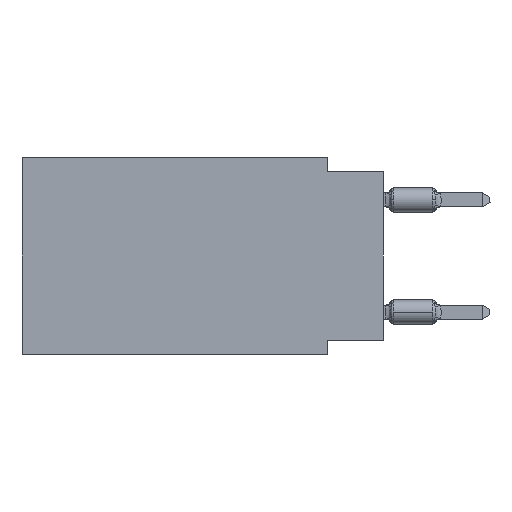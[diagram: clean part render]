
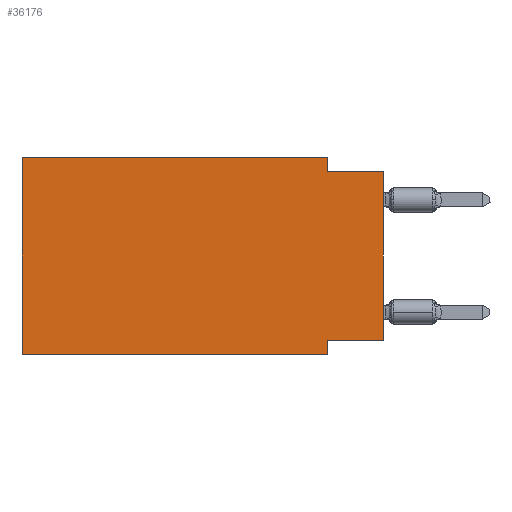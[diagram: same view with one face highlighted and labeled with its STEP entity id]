
A CAD part, left-side view. The second image highlights one B-rep face of the part: STEP entity #36176.
In plain terms, the highlighted planar face has unit normal (-1, 0, 0).
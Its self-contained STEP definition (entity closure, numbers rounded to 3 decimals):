
#5081 = CARTESIAN_POINT ( 'NONE',  ( 0., 0., -0.635 ) ) ;
#5878 = LINE ( 'NONE', #24219, #39265 ) ;
#6838 = VECTOR ( 'NONE', #38249, 1000. ) ;
#7931 = CARTESIAN_POINT ( 'NONE',  ( 0., 2.54, 0. ) ) ;
#9009 = EDGE_CURVE ( 'NONE', #35786, #32099, #42943, .T. ) ;
#9018 = VECTOR ( 'NONE', #39912, 1000. ) ;
#9441 = VERTEX_POINT ( 'NONE', #12485 ) ;
#9803 = AXIS2_PLACEMENT_3D ( 'NONE', #36194, #58762, #30806 ) ;
#11389 = DIRECTION ( 'NONE',  ( 0., 0., 1. ) ) ;
#11688 = CARTESIAN_POINT ( 'NONE',  ( 0., 0., -8.255 ) ) ;
#12299 = ORIENTED_EDGE ( 'NONE', *, *, #9009, .T. ) ;
#12485 = CARTESIAN_POINT ( 'NONE',  ( 0., 2.54, -0.635 ) ) ;
#12638 = CARTESIAN_POINT ( 'NONE',  ( 0., 0., -8.255 ) ) ;
#14090 = EDGE_CURVE ( 'NONE', #54778, #34533, #27124, .T. ) ;
#14154 = EDGE_CURVE ( 'NONE', #33876, #26621, #50866, .T. ) ;
#15333 = CARTESIAN_POINT ( 'NONE',  ( 0., 2.54, -8.89 ) ) ;
#15729 = VECTOR ( 'NONE', #11389, 1000. ) ;
#15872 = VECTOR ( 'NONE', #42698, 1000. ) ;
#16731 = EDGE_CURVE ( 'NONE', #40466, #9441, #20872, .T. ) ;
#17836 = EDGE_CURVE ( 'NONE', #26621, #40466, #5878, .T. ) ;
#18062 = VECTOR ( 'NONE', #42431, 1000. ) ;
#18704 = EDGE_CURVE ( 'NONE', #33876, #34533, #46908, .T. ) ;
#19930 = CARTESIAN_POINT ( 'NONE',  ( 0., 0., -0.635 ) ) ;
#20116 = CARTESIAN_POINT ( 'NONE',  ( 0., 0., 0. ) ) ;
#20848 = ORIENTED_EDGE ( 'NONE', *, *, #53926, .F. ) ;
#20872 = LINE ( 'NONE', #7931, #47003 ) ;
#21926 = ORIENTED_EDGE ( 'NONE', *, *, #45722, .F. ) ;
#22688 = CARTESIAN_POINT ( 'NONE',  ( 0., 2.54, -8.255 ) ) ;
#24219 = CARTESIAN_POINT ( 'NONE',  ( 0., 16.383, 0. ) ) ;
#25162 = ORIENTED_EDGE ( 'NONE', *, *, #14090, .F. ) ;
#26089 = ORIENTED_EDGE ( 'NONE', *, *, #17836, .F. ) ;
#26518 = CARTESIAN_POINT ( 'NONE',  ( 0., 2.54, -8.89 ) ) ;
#26621 = VERTEX_POINT ( 'NONE', #32215 ) ;
#27124 = LINE ( 'NONE', #26518, #52612 ) ;
#29075 = ORIENTED_EDGE ( 'NONE', *, *, #16731, .F. ) ;
#30806 = DIRECTION ( 'NONE',  ( 0., 0., -1. ) ) ;
#31397 = PLANE ( 'NONE',  #9803 ) ;
#32099 = VERTEX_POINT ( 'NONE', #5081 ) ;
#32215 = CARTESIAN_POINT ( 'NONE',  ( 0., 16.383, 0. ) ) ;
#33876 = VERTEX_POINT ( 'NONE', #42848 ) ;
#34533 = VERTEX_POINT ( 'NONE', #15333 ) ;
#35786 = VERTEX_POINT ( 'NONE', #12638 ) ;
#36176 = ADVANCED_FACE ( 'NONE', ( #44918 ), #31397, .F. ) ;
#36194 = CARTESIAN_POINT ( 'NONE',  ( 0., 16.383, 0. ) ) ;
#36410 = DIRECTION ( 'NONE',  ( 0., 0., -1. ) ) ;
#37043 = ORIENTED_EDGE ( 'NONE', *, *, #18704, .T. ) ;
#37925 = CARTESIAN_POINT ( 'NONE',  ( 0., 16.383, 0. ) ) ;
#38249 = DIRECTION ( 'NONE',  ( 0., -1., 0. ) ) ;
#39265 = VECTOR ( 'NONE', #55766, 1000. ) ;
#39912 = DIRECTION ( 'NONE',  ( 0., 1., 0. ) ) ;
#40466 = VERTEX_POINT ( 'NONE', #43774 ) ;
#42392 = CARTESIAN_POINT ( 'NONE',  ( 0., 16.383, -8.89 ) ) ;
#42431 = DIRECTION ( 'NONE',  ( 0., 0., 1. ) ) ;
#42698 = DIRECTION ( 'NONE',  ( 0., -1., 0. ) ) ;
#42848 = CARTESIAN_POINT ( 'NONE',  ( 0., 16.383, -8.89 ) ) ;
#42943 = LINE ( 'NONE', #20116, #15729 ) ;
#43774 = CARTESIAN_POINT ( 'NONE',  ( 0., 2.54, 0. ) ) ;
#43991 = DIRECTION ( 'NONE',  ( 0., 0., -1. ) ) ;
#44918 = FACE_OUTER_BOUND ( 'NONE', #51014, .T. ) ;
#45722 = EDGE_CURVE ( 'NONE', #9441, #32099, #51498, .T. ) ;
#46908 = LINE ( 'NONE', #42392, #15872 ) ;
#47003 = VECTOR ( 'NONE', #43991, 1000. ) ;
#50176 = ORIENTED_EDGE ( 'NONE', *, *, #14154, .F. ) ;
#50866 = LINE ( 'NONE', #37925, #18062 ) ;
#51014 = EDGE_LOOP ( 'NONE', ( #12299, #21926, #29075, #26089, #50176, #37043, #25162, #20848 ) ) ;
#51498 = LINE ( 'NONE', #19930, #6838 ) ;
#52612 = VECTOR ( 'NONE', #36410, 1000. ) ;
#53926 = EDGE_CURVE ( 'NONE', #35786, #54778, #58547, .T. ) ;
#54778 = VERTEX_POINT ( 'NONE', #22688 ) ;
#55766 = DIRECTION ( 'NONE',  ( 0., -1., 0. ) ) ;
#58547 = LINE ( 'NONE', #11688, #9018 ) ;
#58762 = DIRECTION ( 'NONE',  ( 1., 0., 0. ) ) ;
